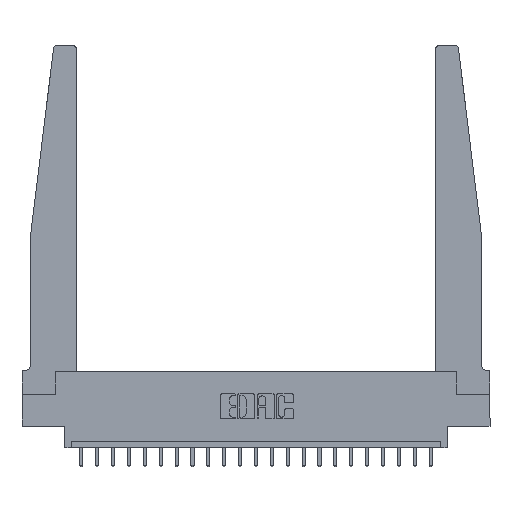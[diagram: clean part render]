
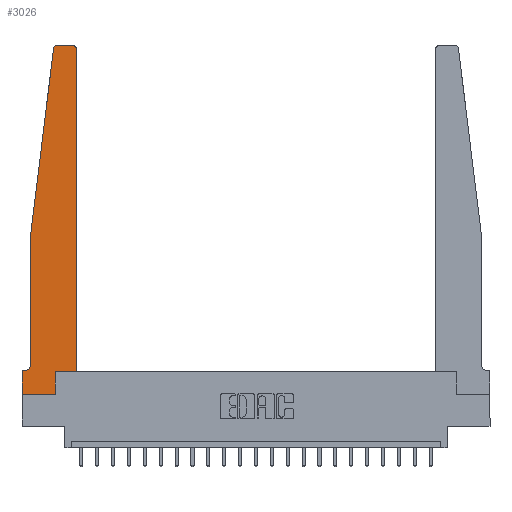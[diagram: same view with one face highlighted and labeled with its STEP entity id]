
A CAD part, top view. The second image highlights one B-rep face of the part: STEP entity #3026.
In plain terms, the highlighted planar face has unit normal (0, 0, 1).
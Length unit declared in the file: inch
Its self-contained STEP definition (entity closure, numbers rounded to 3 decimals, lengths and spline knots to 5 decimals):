
#53 = CARTESIAN_POINT ( 'NONE',  ( 0.2605, 0., 0.37 ) ) ;
#610 = CARTESIAN_POINT ( 'NONE',  ( 0., 0.1875, 0.37 ) ) ;
#919 = AXIS2_PLACEMENT_3D ( 'NONE', #4591, #16182, #12836 ) ;
#1064 = ORIENTED_EDGE ( 'NONE', *, *, #17472, .T. ) ;
#1290 = CARTESIAN_POINT ( 'NONE',  ( 0.065, 1.25, 0.37 ) ) ;
#1576 = CARTESIAN_POINT ( 'NONE',  ( 0.425, 2.72, 0.37 ) ) ;
#1868 = CIRCLE ( 'NONE', #5731, 0.05 ) ;
#1924 = CARTESIAN_POINT ( 'NONE',  ( 0.065, 1.25, 0.37 ) ) ;
#2007 = ORIENTED_EDGE ( 'NONE', *, *, #16655, .T. ) ;
#2603 = CIRCLE ( 'NONE', #9794, 0.03 ) ;
#3026 = ADVANCED_FACE ( 'NONE', ( #6885 ), #9418, .T. ) ;
#3083 = LINE ( 'NONE', #12503, #17821 ) ;
#3134 = CARTESIAN_POINT ( 'NONE',  ( 0.24675, 2.72367, 0.37 ) ) ;
#3203 = LINE ( 'NONE', #1924, #6327 ) ;
#3469 = DIRECTION ( 'NONE',  ( 0., -1., 0. ) ) ;
#3606 = VERTEX_POINT ( 'NONE', #14677 ) ;
#3732 = VECTOR ( 'NONE', #14773, 39.37008 ) ;
#3856 = ORIENTED_EDGE ( 'NONE', *, *, #11704, .T. ) ;
#4246 = DIRECTION ( 'NONE',  ( -1., 0., 0. ) ) ;
#4401 = DIRECTION ( 'NONE',  ( -0.122, -0.992, 0. ) ) ;
#4591 = CARTESIAN_POINT ( 'NONE',  ( 0., 0.1875, 0.37 ) ) ;
#4802 = CARTESIAN_POINT ( 'NONE',  ( 0.425, 0.18, 0.37 ) ) ;
#4827 = CARTESIAN_POINT ( 'NONE',  ( 0.2605, 0.18, 0.37 ) ) ;
#5358 = DIRECTION ( 'NONE',  ( 1., 0., 0. ) ) ;
#5476 = LINE ( 'NONE', #1290, #20529 ) ;
#5497 = DIRECTION ( 'NONE',  ( 0., 0., -1. ) ) ;
#5731 = AXIS2_PLACEMENT_3D ( 'NONE', #10721, #5497, #13858 ) ;
#6050 = ORIENTED_EDGE ( 'NONE', *, *, #7682, .T. ) ;
#6225 = LINE ( 'NONE', #14984, #16561 ) ;
#6272 = CARTESIAN_POINT ( 'NONE',  ( 0.065, 0.2375, 0.37 ) ) ;
#6327 = VECTOR ( 'NONE', #3469, 39.37008 ) ;
#6628 = DIRECTION ( 'NONE',  ( 0., -1., 0. ) ) ;
#6885 = FACE_OUTER_BOUND ( 'NONE', #7194, .T. ) ;
#7041 = DIRECTION ( 'NONE',  ( 1., 0., 0. ) ) ;
#7193 = VECTOR ( 'NONE', #7041, 39.37008 ) ;
#7194 = EDGE_LOOP ( 'NONE', ( #3856, #2007, #7362, #11323, #9120, #18038, #7365, #15474, #19299, #1064, #6050, #14533 ) ) ;
#7332 = VERTEX_POINT ( 'NONE', #16268 ) ;
#7362 = ORIENTED_EDGE ( 'NONE', *, *, #20510, .T. ) ;
#7365 = ORIENTED_EDGE ( 'NONE', *, *, #15082, .T. ) ;
#7393 = EDGE_CURVE ( 'NONE', #17068, #16130, #15306, .T. ) ;
#7428 = DIRECTION ( 'NONE',  ( 0., 0., 1. ) ) ;
#7462 = CIRCLE ( 'NONE', #16444, 0.03 ) ;
#7682 = EDGE_CURVE ( 'NONE', #9071, #17952, #15035, .T. ) ;
#7698 = CARTESIAN_POINT ( 'NONE',  ( 0.425, 0.18, 0.37 ) ) ;
#7866 = EDGE_CURVE ( 'NONE', #11840, #7332, #1868, .T. ) ;
#8444 = LINE ( 'NONE', #11064, #21403 ) ;
#8930 = VECTOR ( 'NONE', #16615, 39.37008 ) ;
#9071 = VERTEX_POINT ( 'NONE', #7698 ) ;
#9120 = ORIENTED_EDGE ( 'NONE', *, *, #7866, .T. ) ;
#9418 = PLANE ( 'NONE',  #919 ) ;
#9631 = EDGE_CURVE ( 'NONE', #16130, #12533, #11959, .T. ) ;
#9700 = VERTEX_POINT ( 'NONE', #3134 ) ;
#9794 = AXIS2_PLACEMENT_3D ( 'NONE', #19286, #7428, #19357 ) ;
#10721 = CARTESIAN_POINT ( 'NONE',  ( 0.015, 0.2375, 0.37 ) ) ;
#10883 = CARTESIAN_POINT ( 'NONE',  ( 0., 0., 0.37 ) ) ;
#11064 = CARTESIAN_POINT ( 'NONE',  ( 0.25, 2.75, 0.37 ) ) ;
#11323 = ORIENTED_EDGE ( 'NONE', *, *, #19627, .T. ) ;
#11409 = CARTESIAN_POINT ( 'NONE',  ( 0.2605, 0.18, 0.37 ) ) ;
#11704 = EDGE_CURVE ( 'NONE', #3606, #16395, #8444, .T. ) ;
#11840 = VERTEX_POINT ( 'NONE', #6272 ) ;
#11959 = LINE ( 'NONE', #11409, #15971 ) ;
#12503 = CARTESIAN_POINT ( 'NONE',  ( 0.065, 0.1875, 0.37 ) ) ;
#12533 = VERTEX_POINT ( 'NONE', #4827 ) ;
#12836 = DIRECTION ( 'NONE',  ( 1., 0., 0. ) ) ;
#13024 = LINE ( 'NONE', #17467, #7193 ) ;
#13638 = CARTESIAN_POINT ( 'NONE',  ( 0.27653, 2.72, 0.37 ) ) ;
#13730 = CARTESIAN_POINT ( 'NONE',  ( 0.065, 1.25, 0.37 ) ) ;
#13858 = DIRECTION ( 'NONE',  ( -1., 0., 0. ) ) ;
#14379 = DIRECTION ( 'NONE',  ( -1., 0., 0. ) ) ;
#14533 = ORIENTED_EDGE ( 'NONE', *, *, #21048, .T. ) ;
#14677 = CARTESIAN_POINT ( 'NONE',  ( 0.395, 2.75, 0.37 ) ) ;
#14773 = DIRECTION ( 'NONE',  ( 1., 0., 0. ) ) ;
#14984 = CARTESIAN_POINT ( 'NONE',  ( 0., 0., 0.37 ) ) ;
#15035 = LINE ( 'NONE', #4802, #8930 ) ;
#15082 = EDGE_CURVE ( 'NONE', #16317, #17068, #6225, .T. ) ;
#15306 = LINE ( 'NONE', #18389, #3732 ) ;
#15474 = ORIENTED_EDGE ( 'NONE', *, *, #7393, .T. ) ;
#15971 = VECTOR ( 'NONE', #17933, 39.37008 ) ;
#16130 = VERTEX_POINT ( 'NONE', #53 ) ;
#16182 = DIRECTION ( 'NONE',  ( 0., 0., 1. ) ) ;
#16268 = CARTESIAN_POINT ( 'NONE',  ( 0.015, 0.1875, 0.37 ) ) ;
#16317 = VERTEX_POINT ( 'NONE', #610 ) ;
#16395 = VERTEX_POINT ( 'NONE', #21184 ) ;
#16444 = AXIS2_PLACEMENT_3D ( 'NONE', #13638, #20645, #5358 ) ;
#16561 = VECTOR ( 'NONE', #6628, 39.37008 ) ;
#16615 = DIRECTION ( 'NONE',  ( 0., 1., 0. ) ) ;
#16655 = EDGE_CURVE ( 'NONE', #16395, #9700, #7462, .T. ) ;
#16794 = EDGE_CURVE ( 'NONE', #7332, #16317, #3083, .T. ) ;
#16921 = VERTEX_POINT ( 'NONE', #13730 ) ;
#17068 = VERTEX_POINT ( 'NONE', #10883 ) ;
#17467 = CARTESIAN_POINT ( 'NONE',  ( 0.425, 0.18, 0.37 ) ) ;
#17472 = EDGE_CURVE ( 'NONE', #12533, #9071, #13024, .T. ) ;
#17821 = VECTOR ( 'NONE', #14379, 39.37008 ) ;
#17933 = DIRECTION ( 'NONE',  ( 0., 1., 0. ) ) ;
#17952 = VERTEX_POINT ( 'NONE', #1576 ) ;
#18038 = ORIENTED_EDGE ( 'NONE', *, *, #16794, .T. ) ;
#18389 = CARTESIAN_POINT ( 'NONE',  ( 0., 0., 0.37 ) ) ;
#19286 = CARTESIAN_POINT ( 'NONE',  ( 0.395, 2.72, 0.37 ) ) ;
#19299 = ORIENTED_EDGE ( 'NONE', *, *, #9631, .T. ) ;
#19357 = DIRECTION ( 'NONE',  ( 1., 0., 0. ) ) ;
#19627 = EDGE_CURVE ( 'NONE', #16921, #11840, #3203, .T. ) ;
#20510 = EDGE_CURVE ( 'NONE', #9700, #16921, #5476, .T. ) ;
#20529 = VECTOR ( 'NONE', #4401, 39.37008 ) ;
#20645 = DIRECTION ( 'NONE',  ( 0., 0., 1. ) ) ;
#21048 = EDGE_CURVE ( 'NONE', #17952, #3606, #2603, .T. ) ;
#21184 = CARTESIAN_POINT ( 'NONE',  ( 0.27653, 2.75, 0.37 ) ) ;
#21403 = VECTOR ( 'NONE', #4246, 39.37008 ) ;
